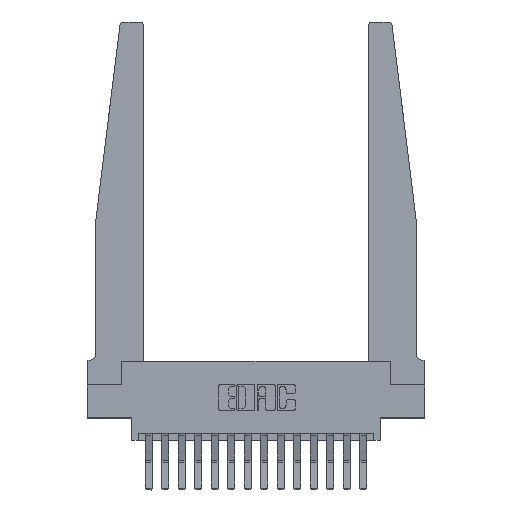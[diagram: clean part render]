
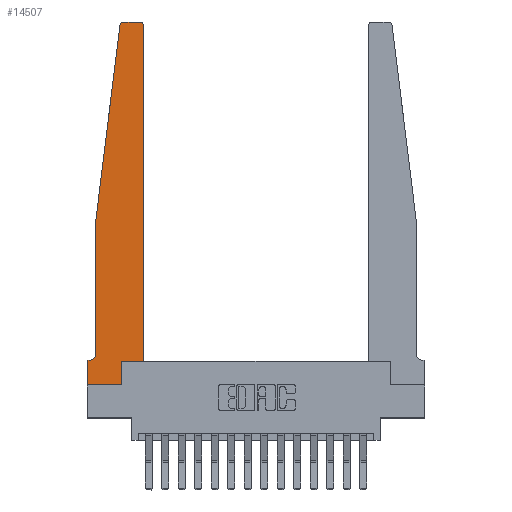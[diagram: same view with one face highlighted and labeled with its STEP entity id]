
A CAD part, top view. The second image highlights one B-rep face of the part: STEP entity #14507.
In plain terms, the highlighted planar face has unit normal (0, 0, 1).
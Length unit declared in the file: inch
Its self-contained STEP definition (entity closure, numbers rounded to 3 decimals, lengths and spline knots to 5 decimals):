
#44 = CARTESIAN_POINT ( 'NONE',  ( 0.015, 0.2375, 0.37 ) ) ;
#122 = EDGE_CURVE ( 'NONE', #6719, #775, #11692, .T. ) ;
#309 = EDGE_CURVE ( 'NONE', #15589, #5049, #9106, .T. ) ;
#350 = CARTESIAN_POINT ( 'NONE',  ( 0., 0., 0.37 ) ) ;
#449 = LINE ( 'NONE', #350, #3661 ) ;
#463 = VECTOR ( 'NONE', #4193, 39.37008 ) ;
#707 = ORIENTED_EDGE ( 'NONE', *, *, #17410, .T. ) ;
#775 = VERTEX_POINT ( 'NONE', #2130 ) ;
#864 = VERTEX_POINT ( 'NONE', #12041 ) ;
#979 = DIRECTION ( 'NONE',  ( -1., 0., 0. ) ) ;
#1019 = CARTESIAN_POINT ( 'NONE',  ( 0., 0.1875, 0.37 ) ) ;
#1416 = DIRECTION ( 'NONE',  ( -1., 0., 0. ) ) ;
#1690 = VECTOR ( 'NONE', #979, 39.37008 ) ;
#1718 = DIRECTION ( 'NONE',  ( 1., 0., 0. ) ) ;
#2056 = AXIS2_PLACEMENT_3D ( 'NONE', #17403, #10654, #17898 ) ;
#2073 = VECTOR ( 'NONE', #12637, 39.37008 ) ;
#2130 = CARTESIAN_POINT ( 'NONE',  ( 0.24675, 2.72367, 0.37 ) ) ;
#2276 = CARTESIAN_POINT ( 'NONE',  ( 0.425, 0.18, 0.37 ) ) ;
#2365 = LINE ( 'NONE', #17023, #12961 ) ;
#2449 = ORIENTED_EDGE ( 'NONE', *, *, #8342, .T. ) ;
#2756 = EDGE_CURVE ( 'NONE', #17074, #9816, #6619, .T. ) ;
#2832 = CARTESIAN_POINT ( 'NONE',  ( 0.25, 2.75, 0.37 ) ) ;
#2945 = VERTEX_POINT ( 'NONE', #7489 ) ;
#3146 = LINE ( 'NONE', #6647, #14156 ) ;
#3464 = ORIENTED_EDGE ( 'NONE', *, *, #16620, .T. ) ;
#3525 = AXIS2_PLACEMENT_3D ( 'NONE', #1019, #7961, #17639 ) ;
#3661 = VECTOR ( 'NONE', #1718, 39.37008 ) ;
#3933 = LINE ( 'NONE', #8985, #17367 ) ;
#4193 = DIRECTION ( 'NONE',  ( -1., 0., 0. ) ) ;
#4407 = CARTESIAN_POINT ( 'NONE',  ( 0.065, 1.25, 0.37 ) ) ;
#4612 = ORIENTED_EDGE ( 'NONE', *, *, #309, .T. ) ;
#4961 = LINE ( 'NONE', #2832, #463 ) ;
#5049 = VERTEX_POINT ( 'NONE', #2276 ) ;
#5065 = ORIENTED_EDGE ( 'NONE', *, *, #13989, .T. ) ;
#5402 = CARTESIAN_POINT ( 'NONE',  ( 0.425, 0.18, 0.37 ) ) ;
#5963 = CARTESIAN_POINT ( 'NONE',  ( 0.395, 2.75, 0.37 ) ) ;
#6427 = AXIS2_PLACEMENT_3D ( 'NONE', #44, #9722, #1416 ) ;
#6559 = PLANE ( 'NONE',  #3525 ) ;
#6619 = LINE ( 'NONE', #8489, #2073 ) ;
#6647 = CARTESIAN_POINT ( 'NONE',  ( 0.065, 1.25, 0.37 ) ) ;
#6697 = CIRCLE ( 'NONE', #6427, 0.05 ) ;
#6719 = VERTEX_POINT ( 'NONE', #7935 ) ;
#6773 = EDGE_CURVE ( 'NONE', #775, #17074, #3146, .T. ) ;
#6955 = ORIENTED_EDGE ( 'NONE', *, *, #15956, .T. ) ;
#7489 = CARTESIAN_POINT ( 'NONE',  ( 0.425, 2.72, 0.37 ) ) ;
#7583 = DIRECTION ( 'NONE',  ( 0., 0., 1. ) ) ;
#7935 = CARTESIAN_POINT ( 'NONE',  ( 0.27653, 2.75, 0.37 ) ) ;
#7961 = DIRECTION ( 'NONE',  ( 0., 0., 1. ) ) ;
#8342 = EDGE_CURVE ( 'NONE', #11290, #15589, #16524, .T. ) ;
#8489 = CARTESIAN_POINT ( 'NONE',  ( 0.065, 1.25, 0.37 ) ) ;
#8632 = LINE ( 'NONE', #9262, #1690 ) ;
#8658 = AXIS2_PLACEMENT_3D ( 'NONE', #15884, #7583, #17270 ) ;
#8676 = VECTOR ( 'NONE', #15099, 39.37008 ) ;
#8900 = ORIENTED_EDGE ( 'NONE', *, *, #16094, .T. ) ;
#8985 = CARTESIAN_POINT ( 'NONE',  ( 0., 0., 0.37 ) ) ;
#9096 = DIRECTION ( 'NONE',  ( 0., 1., 0. ) ) ;
#9106 = LINE ( 'NONE', #5402, #8676 ) ;
#9262 = CARTESIAN_POINT ( 'NONE',  ( 0.065, 0.1875, 0.37 ) ) ;
#9540 = ORIENTED_EDGE ( 'NONE', *, *, #16511, .T. ) ;
#9722 = DIRECTION ( 'NONE',  ( 0., 0., -1. ) ) ;
#9816 = VERTEX_POINT ( 'NONE', #9965 ) ;
#9965 = CARTESIAN_POINT ( 'NONE',  ( 0.065, 0.2375, 0.37 ) ) ;
#10250 = DIRECTION ( 'NONE',  ( 0., 1., 0. ) ) ;
#10370 = DIRECTION ( 'NONE',  ( 0., -1., 0. ) ) ;
#10606 = VERTEX_POINT ( 'NONE', #11673 ) ;
#10654 = DIRECTION ( 'NONE',  ( 0., 0., 1. ) ) ;
#11290 = VERTEX_POINT ( 'NONE', #12015 ) ;
#11673 = CARTESIAN_POINT ( 'NONE',  ( 0., 0., 0.37 ) ) ;
#11692 = CIRCLE ( 'NONE', #2056, 0.03 ) ;
#12015 = CARTESIAN_POINT ( 'NONE',  ( 0.2605, 0., 0.37 ) ) ;
#12041 = CARTESIAN_POINT ( 'NONE',  ( 0.015, 0.1875, 0.37 ) ) ;
#12071 = ORIENTED_EDGE ( 'NONE', *, *, #6773, .T. ) ;
#12637 = DIRECTION ( 'NONE',  ( 0., -1., 0. ) ) ;
#12758 = CARTESIAN_POINT ( 'NONE',  ( 0., 0.1875, 0.37 ) ) ;
#12787 = EDGE_LOOP ( 'NONE', ( #6955, #17183, #12071, #14591, #16829, #707, #5065, #9540, #2449, #4612, #3464, #8900 ) ) ;
#12961 = VECTOR ( 'NONE', #10250, 39.37008 ) ;
#13647 = FACE_OUTER_BOUND ( 'NONE', #12787, .T. ) ;
#13683 = VECTOR ( 'NONE', #9096, 39.37008 ) ;
#13989 = EDGE_CURVE ( 'NONE', #17114, #10606, #3933, .T. ) ;
#14156 = VECTOR ( 'NONE', #16345, 39.37008 ) ;
#14507 = ADVANCED_FACE ( 'NONE', ( #13647 ), #6559, .T. ) ;
#14591 = ORIENTED_EDGE ( 'NONE', *, *, #2756, .T. ) ;
#15099 = DIRECTION ( 'NONE',  ( 1., 0., 0. ) ) ;
#15589 = VERTEX_POINT ( 'NONE', #17177 ) ;
#15884 = CARTESIAN_POINT ( 'NONE',  ( 0.395, 2.72, 0.37 ) ) ;
#15956 = EDGE_CURVE ( 'NONE', #17835, #6719, #4961, .T. ) ;
#16094 = EDGE_CURVE ( 'NONE', #2945, #17835, #17105, .T. ) ;
#16333 = EDGE_CURVE ( 'NONE', #9816, #864, #6697, .T. ) ;
#16345 = DIRECTION ( 'NONE',  ( -0.122, -0.992, 0. ) ) ;
#16511 = EDGE_CURVE ( 'NONE', #10606, #11290, #449, .T. ) ;
#16524 = LINE ( 'NONE', #17377, #13683 ) ;
#16620 = EDGE_CURVE ( 'NONE', #5049, #2945, #2365, .T. ) ;
#16829 = ORIENTED_EDGE ( 'NONE', *, *, #16333, .T. ) ;
#17023 = CARTESIAN_POINT ( 'NONE',  ( 0.425, 0.18, 0.37 ) ) ;
#17074 = VERTEX_POINT ( 'NONE', #4407 ) ;
#17105 = CIRCLE ( 'NONE', #8658, 0.03 ) ;
#17114 = VERTEX_POINT ( 'NONE', #12758 ) ;
#17177 = CARTESIAN_POINT ( 'NONE',  ( 0.2605, 0.18, 0.37 ) ) ;
#17183 = ORIENTED_EDGE ( 'NONE', *, *, #122, .T. ) ;
#17270 = DIRECTION ( 'NONE',  ( 1., 0., 0. ) ) ;
#17367 = VECTOR ( 'NONE', #10370, 39.37008 ) ;
#17377 = CARTESIAN_POINT ( 'NONE',  ( 0.2605, 0.18, 0.37 ) ) ;
#17403 = CARTESIAN_POINT ( 'NONE',  ( 0.27653, 2.72, 0.37 ) ) ;
#17410 = EDGE_CURVE ( 'NONE', #864, #17114, #8632, .T. ) ;
#17639 = DIRECTION ( 'NONE',  ( 1., 0., 0. ) ) ;
#17835 = VERTEX_POINT ( 'NONE', #5963 ) ;
#17898 = DIRECTION ( 'NONE',  ( 1., 0., 0. ) ) ;
